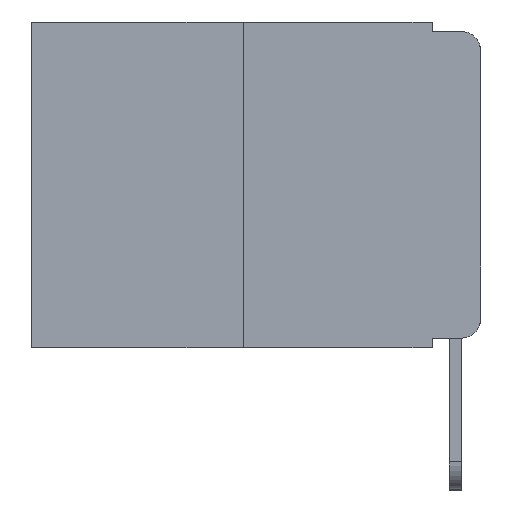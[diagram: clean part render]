
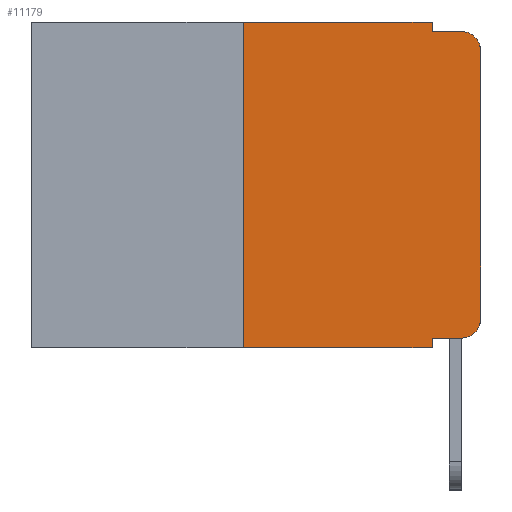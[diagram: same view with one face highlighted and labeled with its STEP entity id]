
A CAD part, left-side view. The second image highlights one B-rep face of the part: STEP entity #11179.
In plain terms, the highlighted planar face has unit normal (-1, 0, 0).
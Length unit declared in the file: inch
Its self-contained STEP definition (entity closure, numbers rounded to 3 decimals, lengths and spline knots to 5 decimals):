
#125 = CARTESIAN_POINT ( 'NONE',  ( 0., 0.02, -0.03 ) ) ;
#340 = EDGE_CURVE ( 'NONE', #5022, #5805, #12284, .T. ) ;
#404 = ORIENTED_EDGE ( 'NONE', *, *, #10069, .F. ) ;
#1081 = DIRECTION ( 'NONE',  ( -1., 0., 0. ) ) ;
#1188 = FACE_OUTER_BOUND ( 'NONE', #5202, .T. ) ;
#1222 = DIRECTION ( 'NONE',  ( 0., 0., -1. ) ) ;
#1276 = VERTEX_POINT ( 'NONE', #8808 ) ;
#1608 = DIRECTION ( 'NONE',  ( 0., -1., 0. ) ) ;
#1683 = DIRECTION ( 'NONE',  ( 0., -1., 0. ) ) ;
#1734 = ORIENTED_EDGE ( 'NONE', *, *, #12185, .F. ) ;
#1780 = ORIENTED_EDGE ( 'NONE', *, *, #5851, .T. ) ;
#2125 = VECTOR ( 'NONE', #1608, 39.37008 ) ;
#2233 = DIRECTION ( 'NONE',  ( 0., -1., 0. ) ) ;
#2238 = CARTESIAN_POINT ( 'NONE',  ( 0., 0.051, 0. ) ) ;
#2365 = DIRECTION ( 'NONE',  ( 1., 0., 0. ) ) ;
#2505 = VERTEX_POINT ( 'NONE', #6628 ) ;
#2577 = ORIENTED_EDGE ( 'NONE', *, *, #7914, .T. ) ;
#2648 = LINE ( 'NONE', #3660, #3864 ) ;
#2667 = CARTESIAN_POINT ( 'NONE',  ( 0., 0.051, -0.343 ) ) ;
#2766 = LINE ( 'NONE', #3814, #4740 ) ;
#3278 = PLANE ( 'NONE',  #5175 ) ;
#3625 = CARTESIAN_POINT ( 'NONE',  ( 0., 0.02, -0.313 ) ) ;
#3660 = CARTESIAN_POINT ( 'NONE',  ( 0., 0.25, 0. ) ) ;
#3675 = DIRECTION ( 'NONE',  ( -1., 0., 0. ) ) ;
#3814 = CARTESIAN_POINT ( 'NONE',  ( 0., 0., 0. ) ) ;
#3835 = CARTESIAN_POINT ( 'NONE',  ( 0., 0.051, -0.333 ) ) ;
#3864 = VECTOR ( 'NONE', #9478, 39.37008 ) ;
#4171 = CARTESIAN_POINT ( 'NONE',  ( 0., 0.051, 0. ) ) ;
#4174 = CARTESIAN_POINT ( 'NONE',  ( 0., 0.25, -0.343 ) ) ;
#4366 = AXIS2_PLACEMENT_3D ( 'NONE', #3625, #3675, #7449 ) ;
#4607 = LINE ( 'NONE', #10708, #8338 ) ;
#4648 = EDGE_CURVE ( 'NONE', #9366, #2505, #11887, .T. ) ;
#4740 = VECTOR ( 'NONE', #9498, 39.37008 ) ;
#4972 = VECTOR ( 'NONE', #1222, 39.37008 ) ;
#5022 = VERTEX_POINT ( 'NONE', #4171 ) ;
#5175 = AXIS2_PLACEMENT_3D ( 'NONE', #9981, #2365, #9188 ) ;
#5202 = EDGE_LOOP ( 'NONE', ( #2577, #1780, #9374, #6451, #12277, #1734, #10433, #404, #7371, #12232 ) ) ;
#5273 = LINE ( 'NONE', #11704, #4972 ) ;
#5364 = VERTEX_POINT ( 'NONE', #2667 ) ;
#5413 = CARTESIAN_POINT ( 'NONE',  ( 0., 0.051, -0.01 ) ) ;
#5467 = EDGE_CURVE ( 'NONE', #11499, #5022, #11567, .T. ) ;
#5688 = VECTOR ( 'NONE', #2233, 39.37008 ) ;
#5805 = VERTEX_POINT ( 'NONE', #5413 ) ;
#5851 = EDGE_CURVE ( 'NONE', #1276, #12177, #9149, .T. ) ;
#5866 = CIRCLE ( 'NONE', #4366, 0.02 ) ;
#6093 = AXIS2_PLACEMENT_3D ( 'NONE', #125, #1081, #7806 ) ;
#6399 = CARTESIAN_POINT ( 'NONE',  ( 0., 0., -0.313 ) ) ;
#6411 = EDGE_CURVE ( 'NONE', #11077, #5364, #8947, .T. ) ;
#6451 = ORIENTED_EDGE ( 'NONE', *, *, #340, .F. ) ;
#6628 = CARTESIAN_POINT ( 'NONE',  ( 0., 0.02, -0.333 ) ) ;
#6934 = CARTESIAN_POINT ( 'NONE',  ( 0., 0.25, 0. ) ) ;
#7045 = EDGE_CURVE ( 'NONE', #5805, #12177, #4607, .T. ) ;
#7371 = ORIENTED_EDGE ( 'NONE', *, *, #4648, .T. ) ;
#7449 = DIRECTION ( 'NONE',  ( 0., 0., -1. ) ) ;
#7454 = CARTESIAN_POINT ( 'NONE',  ( 0., 0.051, -0.333 ) ) ;
#7458 = CARTESIAN_POINT ( 'NONE',  ( 0., 0.473, 0. ) ) ;
#7478 = CARTESIAN_POINT ( 'NONE',  ( 0., 0.02, -0.01 ) ) ;
#7801 = VECTOR ( 'NONE', #8935, 39.37008 ) ;
#7806 = DIRECTION ( 'NONE',  ( 0., 0., -1. ) ) ;
#7914 = EDGE_CURVE ( 'NONE', #9328, #1276, #2766, .T. ) ;
#7976 = CARTESIAN_POINT ( 'NONE',  ( 0., 0.473, -0.343 ) ) ;
#8338 = VECTOR ( 'NONE', #11702, 39.37008 ) ;
#8808 = CARTESIAN_POINT ( 'NONE',  ( 0., 0., -0.03 ) ) ;
#8935 = DIRECTION ( 'NONE',  ( 0., 0., -1. ) ) ;
#8947 = LINE ( 'NONE', #7976, #5688 ) ;
#9019 = VECTOR ( 'NONE', #1683, 39.37008 ) ;
#9149 = CIRCLE ( 'NONE', #6093, 0.02 ) ;
#9188 = DIRECTION ( 'NONE',  ( 0., 0., -1. ) ) ;
#9328 = VERTEX_POINT ( 'NONE', #6399 ) ;
#9366 = VERTEX_POINT ( 'NONE', #3835 ) ;
#9374 = ORIENTED_EDGE ( 'NONE', *, *, #7045, .F. ) ;
#9478 = DIRECTION ( 'NONE',  ( 0., 0., 1. ) ) ;
#9498 = DIRECTION ( 'NONE',  ( 0., 0., 1. ) ) ;
#9981 = CARTESIAN_POINT ( 'NONE',  ( 0., 0.473, 0. ) ) ;
#10069 = EDGE_CURVE ( 'NONE', #9366, #5364, #5273, .T. ) ;
#10433 = ORIENTED_EDGE ( 'NONE', *, *, #6411, .T. ) ;
#10708 = CARTESIAN_POINT ( 'NONE',  ( 0., 0.051, -0.01 ) ) ;
#10777 = EDGE_CURVE ( 'NONE', #2505, #9328, #5866, .T. ) ;
#11077 = VERTEX_POINT ( 'NONE', #4174 ) ;
#11179 = ADVANCED_FACE ( 'NONE', ( #1188 ), #3278, .F. ) ;
#11499 = VERTEX_POINT ( 'NONE', #6934 ) ;
#11567 = LINE ( 'NONE', #7458, #2125 ) ;
#11702 = DIRECTION ( 'NONE',  ( 0., -1., 0. ) ) ;
#11704 = CARTESIAN_POINT ( 'NONE',  ( 0., 0.051, 0. ) ) ;
#11887 = LINE ( 'NONE', #7454, #9019 ) ;
#12177 = VERTEX_POINT ( 'NONE', #7478 ) ;
#12185 = EDGE_CURVE ( 'NONE', #11077, #11499, #2648, .T. ) ;
#12232 = ORIENTED_EDGE ( 'NONE', *, *, #10777, .T. ) ;
#12277 = ORIENTED_EDGE ( 'NONE', *, *, #5467, .F. ) ;
#12284 = LINE ( 'NONE', #2238, #7801 ) ;
